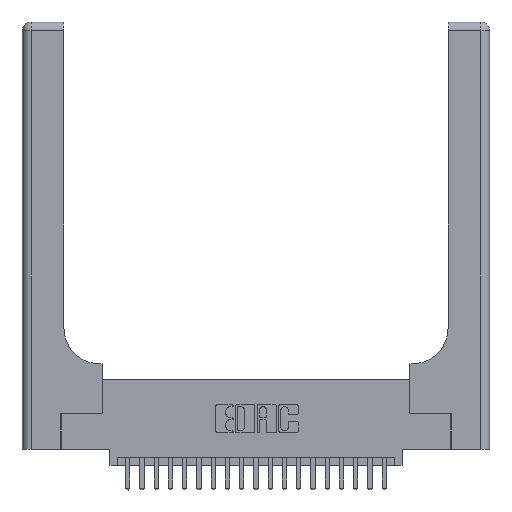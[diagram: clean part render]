
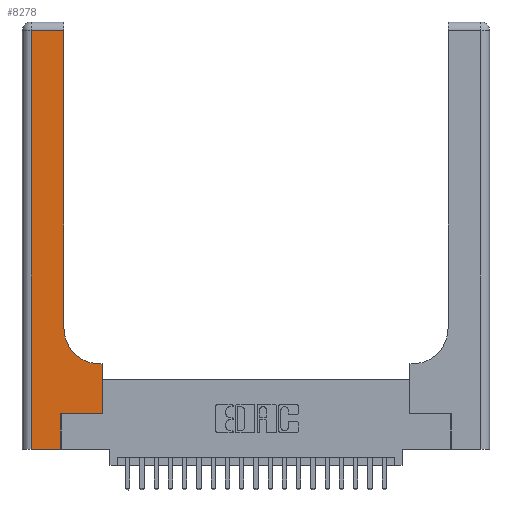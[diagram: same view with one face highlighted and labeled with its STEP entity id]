
A CAD part, top view. The second image highlights one B-rep face of the part: STEP entity #8278.
In plain terms, the highlighted planar face has unit normal (0, 0, 1).
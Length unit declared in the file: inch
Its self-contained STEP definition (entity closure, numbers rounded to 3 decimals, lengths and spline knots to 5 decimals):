
#432 = DIRECTION ( 'NONE',  ( -1., 0., 0. ) ) ;
#473 = VECTOR ( 'NONE', #11872, 39.37008 ) ;
#589 = EDGE_CURVE ( 'NONE', #9959, #6436, #16663, .T. ) ;
#1352 = CARTESIAN_POINT ( 'NONE',  ( 0.2915, 3., 0.37 ) ) ;
#2172 = EDGE_CURVE ( 'NONE', #21270, #4402, #3077, .T. ) ;
#2478 = ORIENTED_EDGE ( 'NONE', *, *, #10704, .T. ) ;
#2908 = EDGE_CURVE ( 'NONE', #6436, #9924, #18011, .T. ) ;
#3077 = LINE ( 'NONE', #22665, #7287 ) ;
#3419 = VERTEX_POINT ( 'NONE', #8195 ) ;
#3425 = CARTESIAN_POINT ( 'NONE',  ( 0.5585, 0.25, 0.37 ) ) ;
#3878 = CARTESIAN_POINT ( 'NONE',  ( 0.5415, 0.6, 0.37 ) ) ;
#4009 = CARTESIAN_POINT ( 'NONE',  ( 0.269, 0., 0.37 ) ) ;
#4315 = EDGE_CURVE ( 'NONE', #5577, #9959, #4904, .T. ) ;
#4402 = VERTEX_POINT ( 'NONE', #3878 ) ;
#4632 = CARTESIAN_POINT ( 'NONE',  ( 0.5585, 0.25, 0.37 ) ) ;
#4728 = VECTOR ( 'NONE', #18695, 39.37008 ) ;
#4904 = LINE ( 'NONE', #1352, #16807 ) ;
#4943 = ORIENTED_EDGE ( 'NONE', *, *, #16995, .T. ) ;
#5577 = VERTEX_POINT ( 'NONE', #17457 ) ;
#5597 = ORIENTED_EDGE ( 'NONE', *, *, #2172, .T. ) ;
#5600 = DIRECTION ( 'NONE',  ( 0., 1., 0. ) ) ;
#6436 = VERTEX_POINT ( 'NONE', #19611 ) ;
#6545 = CARTESIAN_POINT ( 'NONE',  ( 0., 0., 0.37 ) ) ;
#6615 = AXIS2_PLACEMENT_3D ( 'NONE', #20122, #16550, #432 ) ;
#7287 = VECTOR ( 'NONE', #8155, 39.37008 ) ;
#8155 = DIRECTION ( 'NONE',  ( -1., 0., 0. ) ) ;
#8167 = VECTOR ( 'NONE', #22305, 39.37008 ) ;
#8195 = CARTESIAN_POINT ( 'NONE',  ( 0.269, 0.25, 0.37 ) ) ;
#8278 = ADVANCED_FACE ( 'NONE', ( #18696 ), #8903, .F. ) ;
#8740 = ORIENTED_EDGE ( 'NONE', *, *, #21552, .T. ) ;
#8788 = ORIENTED_EDGE ( 'NONE', *, *, #20822, .T. ) ;
#8903 = PLANE ( 'NONE',  #6615 ) ;
#8992 = VECTOR ( 'NONE', #19682, 39.37008 ) ;
#9152 = VERTEX_POINT ( 'NONE', #4632 ) ;
#9368 = VERTEX_POINT ( 'NONE', #4009 ) ;
#9924 = VERTEX_POINT ( 'NONE', #23399 ) ;
#9959 = VERTEX_POINT ( 'NONE', #21821 ) ;
#10660 = CARTESIAN_POINT ( 'NONE',  ( 0.5415, 0.85, 0.37 ) ) ;
#10704 = EDGE_CURVE ( 'NONE', #9924, #9368, #19697, .T. ) ;
#11401 = VECTOR ( 'NONE', #18040, 39.37008 ) ;
#11454 = ORIENTED_EDGE ( 'NONE', *, *, #4315, .T. ) ;
#11872 = DIRECTION ( 'NONE',  ( 1., 0., 0. ) ) ;
#12055 = CARTESIAN_POINT ( 'NONE',  ( 0.5585, 0.6, 0.37 ) ) ;
#12400 = CIRCLE ( 'NONE', #18118, 0.25 ) ;
#16542 = CARTESIAN_POINT ( 'NONE',  ( 0.269, 0., 0.37 ) ) ;
#16550 = DIRECTION ( 'NONE',  ( 0., 0., -1. ) ) ;
#16663 = LINE ( 'NONE', #18258, #8167 ) ;
#16807 = VECTOR ( 'NONE', #5600, 39.37008 ) ;
#16874 = VECTOR ( 'NONE', #23344, 39.37008 ) ;
#16995 = EDGE_CURVE ( 'NONE', #3419, #9152, #22453, .T. ) ;
#17457 = CARTESIAN_POINT ( 'NONE',  ( 0.2915, 0.85, 0.37 ) ) ;
#17752 = LINE ( 'NONE', #16542, #4728 ) ;
#18011 = LINE ( 'NONE', #21533, #16874 ) ;
#18040 = DIRECTION ( 'NONE',  ( 1., 0., 0. ) ) ;
#18118 = AXIS2_PLACEMENT_3D ( 'NONE', #10660, #19734, #23242 ) ;
#18258 = CARTESIAN_POINT ( 'NONE',  ( 0., 2.94, 0.37 ) ) ;
#18695 = DIRECTION ( 'NONE',  ( 0., 1., 0. ) ) ;
#18696 = FACE_OUTER_BOUND ( 'NONE', #21532, .T. ) ;
#19041 = EDGE_CURVE ( 'NONE', #9368, #3419, #17752, .T. ) ;
#19611 = CARTESIAN_POINT ( 'NONE',  ( 0.06, 2.94, 0.37 ) ) ;
#19682 = DIRECTION ( 'NONE',  ( 0., 1., 0. ) ) ;
#19697 = LINE ( 'NONE', #6545, #473 ) ;
#19734 = DIRECTION ( 'NONE',  ( 0., 0., -1. ) ) ;
#19777 = CARTESIAN_POINT ( 'NONE',  ( 0.269, 0.25, 0.37 ) ) ;
#20122 = CARTESIAN_POINT ( 'NONE',  ( 0., 3., 0.37 ) ) ;
#20605 = LINE ( 'NONE', #3425, #8992 ) ;
#20822 = EDGE_CURVE ( 'NONE', #4402, #5577, #12400, .T. ) ;
#21270 = VERTEX_POINT ( 'NONE', #12055 ) ;
#21465 = ORIENTED_EDGE ( 'NONE', *, *, #19041, .T. ) ;
#21532 = EDGE_LOOP ( 'NONE', ( #11454, #22156, #23237, #2478, #21465, #4943, #8740, #5597, #8788 ) ) ;
#21533 = CARTESIAN_POINT ( 'NONE',  ( 0.06, 3., 0.37 ) ) ;
#21552 = EDGE_CURVE ( 'NONE', #9152, #21270, #20605, .T. ) ;
#21821 = CARTESIAN_POINT ( 'NONE',  ( 0.2915, 2.94, 0.37 ) ) ;
#22156 = ORIENTED_EDGE ( 'NONE', *, *, #589, .T. ) ;
#22305 = DIRECTION ( 'NONE',  ( -1., 0., 0. ) ) ;
#22453 = LINE ( 'NONE', #19777, #11401 ) ;
#22665 = CARTESIAN_POINT ( 'NONE',  ( 0.2915, 0.6, 0.37 ) ) ;
#23237 = ORIENTED_EDGE ( 'NONE', *, *, #2908, .T. ) ;
#23242 = DIRECTION ( 'NONE',  ( 1., 0., 0. ) ) ;
#23344 = DIRECTION ( 'NONE',  ( 0., -1., 0. ) ) ;
#23399 = CARTESIAN_POINT ( 'NONE',  ( 0.06, 0., 0.37 ) ) ;
